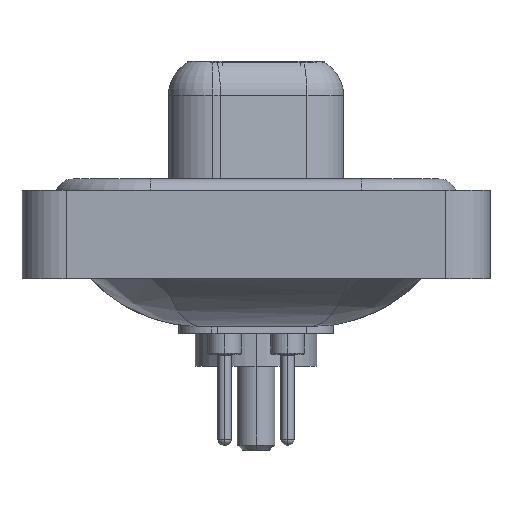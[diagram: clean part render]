
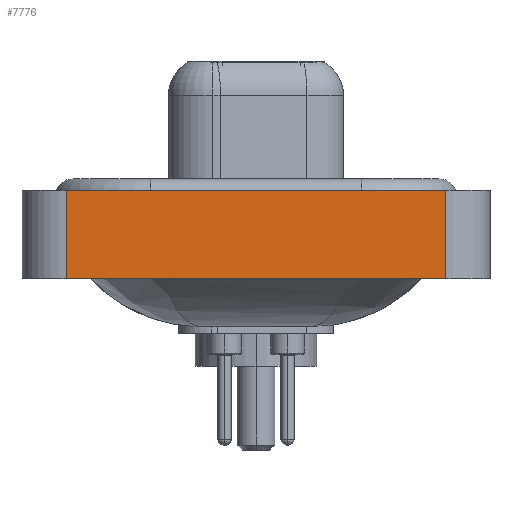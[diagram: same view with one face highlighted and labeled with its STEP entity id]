
A CAD part, left-side view. The second image highlights one B-rep face of the part: STEP entity #7776.
In plain terms, the highlighted planar face has unit normal (-1, 0, 0).
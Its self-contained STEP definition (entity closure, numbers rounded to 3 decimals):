
#219 = VERTEX_POINT ( 'NONE', #7583 ) ;
#597 = CARTESIAN_POINT ( 'NONE',  ( -7.25, 8.55, 0.4 ) ) ;
#673 = DIRECTION ( 'NONE',  ( 0., 0., 1. ) ) ;
#1604 = LINE ( 'NONE', #10791, #18461 ) ;
#2680 = VERTEX_POINT ( 'NONE', #597 ) ;
#4609 = ORIENTED_EDGE ( 'NONE', *, *, #8280, .F. ) ;
#5159 = DIRECTION ( 'NONE',  ( 0., 0., 1. ) ) ;
#5558 = CARTESIAN_POINT ( 'NONE',  ( -7.25, -8.55, 0.4 ) ) ;
#5711 = CARTESIAN_POINT ( 'NONE',  ( -7.25, -8.55, -3.6 ) ) ;
#7583 = CARTESIAN_POINT ( 'NONE',  ( -7.25, -8.55, -3.6 ) ) ;
#7665 = CARTESIAN_POINT ( 'NONE',  ( -7.25, 8.55, -3.6 ) ) ;
#7776 = ADVANCED_FACE ( 'NONE', ( #13236 ), #11845, .T. ) ;
#8280 = EDGE_CURVE ( 'NONE', #2680, #12486, #1604, .T. ) ;
#8355 = ORIENTED_EDGE ( 'NONE', *, *, #10534, .T. ) ;
#8634 = EDGE_CURVE ( 'NONE', #16820, #219, #10764, .T. ) ;
#8997 = DIRECTION ( 'NONE',  ( 0., -1., 0. ) ) ;
#9970 = CARTESIAN_POINT ( 'NONE',  ( -7.25, -8.55, -3.6 ) ) ;
#10534 = EDGE_CURVE ( 'NONE', #219, #12486, #15932, .T. ) ;
#10764 = LINE ( 'NONE', #19505, #15380 ) ;
#10791 = CARTESIAN_POINT ( 'NONE',  ( -7.25, -8.55, 0.4 ) ) ;
#10869 = EDGE_CURVE ( 'NONE', #16820, #2680, #15907, .T. ) ;
#11741 = DIRECTION ( 'NONE',  ( -1., 0., 0. ) ) ;
#11845 = PLANE ( 'NONE',  #15920 ) ;
#11920 = VECTOR ( 'NONE', #673, 1000. ) ;
#12486 = VERTEX_POINT ( 'NONE', #5558 ) ;
#13236 = FACE_OUTER_BOUND ( 'NONE', #14759, .T. ) ;
#14749 = VECTOR ( 'NONE', #5159, 1000. ) ;
#14759 = EDGE_LOOP ( 'NONE', ( #8355, #4609, #16931, #19547 ) ) ;
#15380 = VECTOR ( 'NONE', #8997, 1000. ) ;
#15523 = CARTESIAN_POINT ( 'NONE',  ( -7.25, 8.55, -3.6 ) ) ;
#15907 = LINE ( 'NONE', #15523, #11920 ) ;
#15920 = AXIS2_PLACEMENT_3D ( 'NONE', #5711, #11741, #17775 ) ;
#15932 = LINE ( 'NONE', #9970, #14749 ) ;
#16820 = VERTEX_POINT ( 'NONE', #7665 ) ;
#16851 = DIRECTION ( 'NONE',  ( 0., -1., 0. ) ) ;
#16931 = ORIENTED_EDGE ( 'NONE', *, *, #10869, .F. ) ;
#17775 = DIRECTION ( 'NONE',  ( 0., 0., 1. ) ) ;
#18461 = VECTOR ( 'NONE', #16851, 1000. ) ;
#19505 = CARTESIAN_POINT ( 'NONE',  ( -7.25, -8.55, -3.6 ) ) ;
#19547 = ORIENTED_EDGE ( 'NONE', *, *, #8634, .T. ) ;
